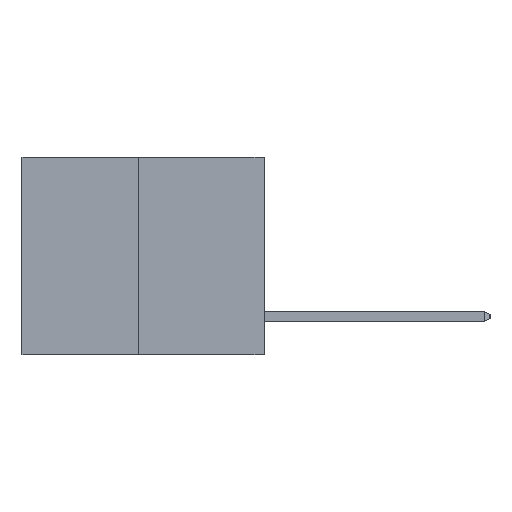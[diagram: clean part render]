
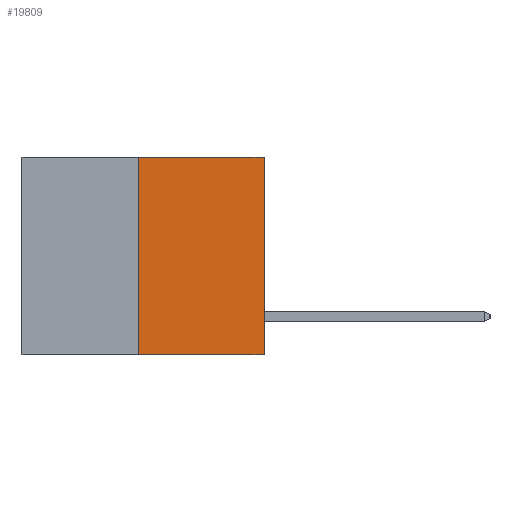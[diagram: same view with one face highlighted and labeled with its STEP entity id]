
A CAD part, left-side view. The second image highlights one B-rep face of the part: STEP entity #19809.
In plain terms, the highlighted planar face has unit normal (-1, 0, 0).
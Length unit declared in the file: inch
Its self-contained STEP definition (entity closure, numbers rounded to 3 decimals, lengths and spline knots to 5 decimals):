
#78 = VECTOR ( 'NONE', #14531, 39.37008 ) ;
#1548 = ORIENTED_EDGE ( 'NONE', *, *, #9765, .T. ) ;
#2172 = CARTESIAN_POINT ( 'NONE',  ( 0., 0.312, -0.49 ) ) ;
#2299 = LINE ( 'NONE', #2172, #9533 ) ;
#2530 = EDGE_LOOP ( 'NONE', ( #4128, #1548, #11639, #6643 ) ) ;
#2885 = CARTESIAN_POINT ( 'NONE',  ( 0., 0., 0. ) ) ;
#3312 = CARTESIAN_POINT ( 'NONE',  ( 0., 0.6, -0.49 ) ) ;
#3670 = VERTEX_POINT ( 'NONE', #2885 ) ;
#4128 = ORIENTED_EDGE ( 'NONE', *, *, #19414, .F. ) ;
#4280 = VERTEX_POINT ( 'NONE', #7213 ) ;
#4845 = DIRECTION ( 'NONE',  ( 0., 0., -1. ) ) ;
#4912 = EDGE_CURVE ( 'NONE', #9813, #3670, #15839, .T. ) ;
#6643 = ORIENTED_EDGE ( 'NONE', *, *, #4912, .F. ) ;
#7213 = CARTESIAN_POINT ( 'NONE',  ( 0., 0., -0.49 ) ) ;
#7525 = CARTESIAN_POINT ( 'NONE',  ( 0., 0.312, -0.49 ) ) ;
#8186 = LINE ( 'NONE', #3312, #14676 ) ;
#8557 = LINE ( 'NONE', #17716, #78 ) ;
#8842 = DIRECTION ( 'NONE',  ( 0., -1., 0. ) ) ;
#9533 = VECTOR ( 'NONE', #11649, 39.37008 ) ;
#9765 = EDGE_CURVE ( 'NONE', #12689, #4280, #8186, .T. ) ;
#9813 = VERTEX_POINT ( 'NONE', #13067 ) ;
#11093 = CARTESIAN_POINT ( 'NONE',  ( 0., 0.6, 0. ) ) ;
#11603 = VECTOR ( 'NONE', #8842, 39.37008 ) ;
#11639 = ORIENTED_EDGE ( 'NONE', *, *, #16408, .T. ) ;
#11649 = DIRECTION ( 'NONE',  ( 0., 0., 1. ) ) ;
#12689 = VERTEX_POINT ( 'NONE', #7525 ) ;
#12763 = FACE_OUTER_BOUND ( 'NONE', #2530, .T. ) ;
#13067 = CARTESIAN_POINT ( 'NONE',  ( 0., 0.312, 0. ) ) ;
#14430 = DIRECTION ( 'NONE',  ( 1., 0., 0. ) ) ;
#14531 = DIRECTION ( 'NONE',  ( 0., 0., 1. ) ) ;
#14676 = VECTOR ( 'NONE', #16064, 39.37008 ) ;
#15279 = CARTESIAN_POINT ( 'NONE',  ( 0., 0.6, 0. ) ) ;
#15839 = LINE ( 'NONE', #15279, #11603 ) ;
#16064 = DIRECTION ( 'NONE',  ( 0., -1., 0. ) ) ;
#16408 = EDGE_CURVE ( 'NONE', #4280, #3670, #8557, .T. ) ;
#16415 = AXIS2_PLACEMENT_3D ( 'NONE', #11093, #14430, #4845 ) ;
#17484 = PLANE ( 'NONE',  #16415 ) ;
#17716 = CARTESIAN_POINT ( 'NONE',  ( 0., 0., 0. ) ) ;
#19414 = EDGE_CURVE ( 'NONE', #12689, #9813, #2299, .T. ) ;
#19809 = ADVANCED_FACE ( 'NONE', ( #12763 ), #17484, .F. ) ;
